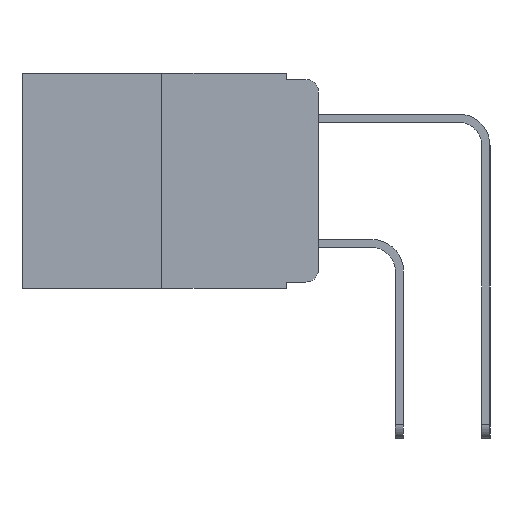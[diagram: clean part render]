
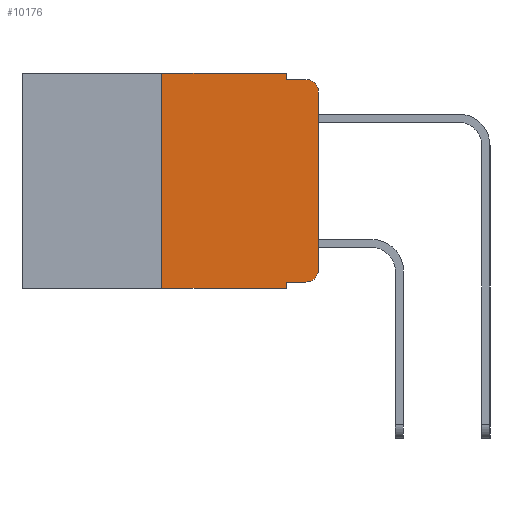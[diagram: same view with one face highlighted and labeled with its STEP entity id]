
A CAD part, left-side view. The second image highlights one B-rep face of the part: STEP entity #10176.
In plain terms, the highlighted planar face has unit normal (-1, 0, 0).
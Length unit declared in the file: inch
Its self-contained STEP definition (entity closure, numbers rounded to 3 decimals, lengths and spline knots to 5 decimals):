
#370 = EDGE_CURVE ( 'NONE', #21779, #8111, #23743, .T. ) ;
#377 = CARTESIAN_POINT ( 'NONE',  ( 0., 0.051, -0.343 ) ) ;
#628 = VECTOR ( 'NONE', #13254, 39.37008 ) ;
#657 = VERTEX_POINT ( 'NONE', #14222 ) ;
#1056 = EDGE_CURVE ( 'NONE', #11356, #22873, #7144, .T. ) ;
#1287 = DIRECTION ( 'NONE',  ( 0., 0., -1. ) ) ;
#1889 = AXIS2_PLACEMENT_3D ( 'NONE', #20107, #7868, #22131 ) ;
#1946 = LINE ( 'NONE', #4385, #23741 ) ;
#2143 = CARTESIAN_POINT ( 'NONE',  ( 0., 0.02, -0.01 ) ) ;
#2268 = DIRECTION ( 'NONE',  ( 0., 0., -1. ) ) ;
#2456 = ORIENTED_EDGE ( 'NONE', *, *, #1056, .T. ) ;
#2673 = CARTESIAN_POINT ( 'NONE',  ( 0., 0.25, 0. ) ) ;
#2909 = ORIENTED_EDGE ( 'NONE', *, *, #24932, .T. ) ;
#3119 = ORIENTED_EDGE ( 'NONE', *, *, #22227, .F. ) ;
#3364 = CARTESIAN_POINT ( 'NONE',  ( 0., 0.473, 0. ) ) ;
#3484 = ORIENTED_EDGE ( 'NONE', *, *, #19537, .F. ) ;
#3573 = ORIENTED_EDGE ( 'NONE', *, *, #370, .F. ) ;
#3753 = ORIENTED_EDGE ( 'NONE', *, *, #16824, .F. ) ;
#3776 = ORIENTED_EDGE ( 'NONE', *, *, #15805, .T. ) ;
#3802 = ORIENTED_EDGE ( 'NONE', *, *, #15445, .F. ) ;
#3911 = VECTOR ( 'NONE', #22250, 39.37008 ) ;
#4129 = ORIENTED_EDGE ( 'NONE', *, *, #14080, .T. ) ;
#4144 = VERTEX_POINT ( 'NONE', #5724 ) ;
#4385 = CARTESIAN_POINT ( 'NONE',  ( 0., 0.051, 0. ) ) ;
#4388 = ORIENTED_EDGE ( 'NONE', *, *, #12710, .T. ) ;
#4608 = EDGE_LOOP ( 'NONE', ( #2456, #2909, #3119, #3484, #3573, #3753, #3776, #3802, #4129, #4388 ) ) ;
#4854 = CARTESIAN_POINT ( 'NONE',  ( 0., 0.25, -0.343 ) ) ;
#5491 = DIRECTION ( 'NONE',  ( 0., 0., -1. ) ) ;
#5724 = CARTESIAN_POINT ( 'NONE',  ( 0., 0.02, -0.333 ) ) ;
#6120 = VECTOR ( 'NONE', #16531, 39.37008 ) ;
#6506 = VECTOR ( 'NONE', #7203, 39.37008 ) ;
#6953 = CIRCLE ( 'NONE', #15535, 0.02 ) ;
#7144 = LINE ( 'NONE', #17434, #6506 ) ;
#7203 = DIRECTION ( 'NONE',  ( 0., 0., 1. ) ) ;
#7498 = VERTEX_POINT ( 'NONE', #25510 ) ;
#7868 = DIRECTION ( 'NONE',  ( -1., 0., 0. ) ) ;
#7973 = VERTEX_POINT ( 'NONE', #377 ) ;
#7992 = CARTESIAN_POINT ( 'NONE',  ( 0., 0.473, -0.343 ) ) ;
#8111 = VERTEX_POINT ( 'NONE', #9212 ) ;
#9212 = CARTESIAN_POINT ( 'NONE',  ( 0., 0.051, 0. ) ) ;
#10013 = VERTEX_POINT ( 'NONE', #4854 ) ;
#10055 = LINE ( 'NONE', #7992, #3911 ) ;
#10176 = ADVANCED_FACE ( 'NONE', ( #14164 ), #25786, .F. ) ;
#10213 = DIRECTION ( 'NONE',  ( 0., -1., 0. ) ) ;
#11356 = VERTEX_POINT ( 'NONE', #21604 ) ;
#11577 = LINE ( 'NONE', #20622, #6120 ) ;
#12703 = VECTOR ( 'NONE', #10213, 39.37008 ) ;
#12710 = EDGE_CURVE ( 'NONE', #4144, #11356, #6953, .T. ) ;
#13254 = DIRECTION ( 'NONE',  ( 0., -1., 0. ) ) ;
#13256 = CARTESIAN_POINT ( 'NONE',  ( 0., 0.25, 0. ) ) ;
#13707 = DIRECTION ( 'NONE',  ( -1., 0., 0. ) ) ;
#13785 = CIRCLE ( 'NONE', #1889, 0.02 ) ;
#13944 = CARTESIAN_POINT ( 'NONE',  ( 0., 0.051, 0. ) ) ;
#14080 = EDGE_CURVE ( 'NONE', #657, #4144, #18138, .T. ) ;
#14164 = FACE_OUTER_BOUND ( 'NONE', #4608, .T. ) ;
#14222 = CARTESIAN_POINT ( 'NONE',  ( 0., 0.051, -0.333 ) ) ;
#14675 = CARTESIAN_POINT ( 'NONE',  ( 0., 0.473, 0. ) ) ;
#15445 = EDGE_CURVE ( 'NONE', #657, #7973, #1946, .T. ) ;
#15535 = AXIS2_PLACEMENT_3D ( 'NONE', #25816, #13707, #1287 ) ;
#15763 = VECTOR ( 'NONE', #21335, 39.37008 ) ;
#15805 = EDGE_CURVE ( 'NONE', #10013, #7973, #10055, .T. ) ;
#16531 = DIRECTION ( 'NONE',  ( 0., -1., 0. ) ) ;
#16586 = VECTOR ( 'NONE', #26111, 39.37008 ) ;
#16824 = EDGE_CURVE ( 'NONE', #10013, #21779, #21796, .T. ) ;
#17434 = CARTESIAN_POINT ( 'NONE',  ( 0., 0., 0. ) ) ;
#17784 = DIRECTION ( 'NONE',  ( 1., 0., 0. ) ) ;
#18138 = LINE ( 'NONE', #18378, #12703 ) ;
#18378 = CARTESIAN_POINT ( 'NONE',  ( 0., 0.051, -0.333 ) ) ;
#19537 = EDGE_CURVE ( 'NONE', #8111, #7498, #22595, .T. ) ;
#19701 = VERTEX_POINT ( 'NONE', #2143 ) ;
#20107 = CARTESIAN_POINT ( 'NONE',  ( 0., 0.02, -0.03 ) ) ;
#20622 = CARTESIAN_POINT ( 'NONE',  ( 0., 0.051, -0.01 ) ) ;
#20948 = CARTESIAN_POINT ( 'NONE',  ( 0., 0., -0.03 ) ) ;
#21335 = DIRECTION ( 'NONE',  ( 0., 0., 1. ) ) ;
#21604 = CARTESIAN_POINT ( 'NONE',  ( 0., 0., -0.313 ) ) ;
#21779 = VERTEX_POINT ( 'NONE', #2673 ) ;
#21796 = LINE ( 'NONE', #13256, #15763 ) ;
#22131 = DIRECTION ( 'NONE',  ( 0., 0., -1. ) ) ;
#22227 = EDGE_CURVE ( 'NONE', #7498, #19701, #11577, .T. ) ;
#22250 = DIRECTION ( 'NONE',  ( 0., -1., 0. ) ) ;
#22595 = LINE ( 'NONE', #13944, #16586 ) ;
#22873 = VERTEX_POINT ( 'NONE', #20948 ) ;
#23741 = VECTOR ( 'NONE', #2268, 39.37008 ) ;
#23743 = LINE ( 'NONE', #14675, #628 ) ;
#24932 = EDGE_CURVE ( 'NONE', #22873, #19701, #13785, .T. ) ;
#24984 = AXIS2_PLACEMENT_3D ( 'NONE', #3364, #17784, #5491 ) ;
#25510 = CARTESIAN_POINT ( 'NONE',  ( 0., 0.051, -0.01 ) ) ;
#25786 = PLANE ( 'NONE',  #24984 ) ;
#25816 = CARTESIAN_POINT ( 'NONE',  ( 0., 0.02, -0.313 ) ) ;
#26111 = DIRECTION ( 'NONE',  ( 0., 0., -1. ) ) ;
